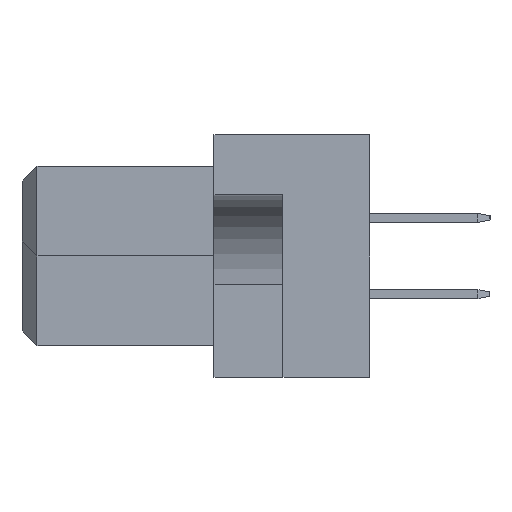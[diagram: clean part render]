
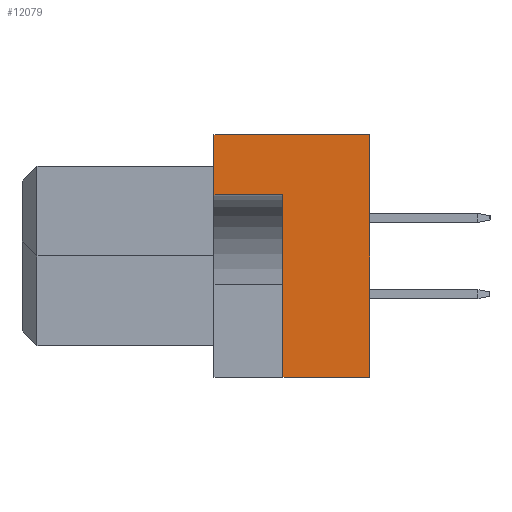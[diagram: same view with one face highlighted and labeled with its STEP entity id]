
A CAD part, left-side view. The second image highlights one B-rep face of the part: STEP entity #12079.
In plain terms, the highlighted planar face has unit normal (-1, 0, 0).
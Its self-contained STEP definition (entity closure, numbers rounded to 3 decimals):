
#908 = ORIENTED_EDGE ( 'NONE', *, *, #6201, .F. ) ;
#1047 = LINE ( 'NONE', #26575, #13743 ) ;
#1635 = VERTEX_POINT ( 'NONE', #16285 ) ;
#1842 = DIRECTION ( 'NONE',  ( 0., -1., 0. ) ) ;
#2089 = CARTESIAN_POINT ( 'NONE',  ( -47.5, 2.9, 2.05 ) ) ;
#2500 = CARTESIAN_POINT ( 'NONE',  ( -47.5, 0., 4.05 ) ) ;
#2769 = VERTEX_POINT ( 'NONE', #9849 ) ;
#2923 = VERTEX_POINT ( 'NONE', #15153 ) ;
#3946 = LINE ( 'NONE', #12339, #15631 ) ;
#4143 = DIRECTION ( 'NONE',  ( 0., 0., -1. ) ) ;
#4178 = DIRECTION ( 'NONE',  ( 0., 0., 1. ) ) ;
#4475 = VERTEX_POINT ( 'NONE', #8277 ) ;
#4609 = LINE ( 'NONE', #2500, #14750 ) ;
#4655 = FACE_OUTER_BOUND ( 'NONE', #23542, .T. ) ;
#6201 = EDGE_CURVE ( 'NONE', #27531, #4475, #25878, .T. ) ;
#6840 = LINE ( 'NONE', #2089, #27155 ) ;
#7661 = AXIS2_PLACEMENT_3D ( 'NONE', #14766, #19911, #4143 ) ;
#7951 = CARTESIAN_POINT ( 'NONE',  ( -47.5, 5.2, 4.05 ) ) ;
#8277 = CARTESIAN_POINT ( 'NONE',  ( -47.5, 0., 4.05 ) ) ;
#9849 = CARTESIAN_POINT ( 'NONE',  ( -47.5, 2.9, 2.05 ) ) ;
#11556 = EDGE_CURVE ( 'NONE', #2923, #27531, #18880, .T. ) ;
#12079 = ADVANCED_FACE ( 'NONE', ( #4655 ), #15290, .F. ) ;
#12339 = CARTESIAN_POINT ( 'NONE',  ( -47.5, 5.2, -4.05 ) ) ;
#13743 = VECTOR ( 'NONE', #15885, 1000. ) ;
#14356 = ORIENTED_EDGE ( 'NONE', *, *, #15703, .T. ) ;
#14566 = ORIENTED_EDGE ( 'NONE', *, *, #15091, .T. ) ;
#14750 = VECTOR ( 'NONE', #21560, 1000. ) ;
#14766 = CARTESIAN_POINT ( 'NONE',  ( -47.5, 5.2, 4.05 ) ) ;
#15091 = EDGE_CURVE ( 'NONE', #1635, #16895, #3946, .T. ) ;
#15153 = CARTESIAN_POINT ( 'NONE',  ( -47.5, 5.2, 2.05 ) ) ;
#15290 = PLANE ( 'NONE',  #7661 ) ;
#15631 = VECTOR ( 'NONE', #1842, 1000. ) ;
#15703 = EDGE_CURVE ( 'NONE', #16895, #4475, #4609, .T. ) ;
#15885 = DIRECTION ( 'NONE',  ( 0., 0., 1. ) ) ;
#16285 = CARTESIAN_POINT ( 'NONE',  ( -47.5, 2.9, -4.05 ) ) ;
#16895 = VERTEX_POINT ( 'NONE', #17355 ) ;
#17355 = CARTESIAN_POINT ( 'NONE',  ( -47.5, 0., -4.05 ) ) ;
#18880 = LINE ( 'NONE', #23360, #22401 ) ;
#19032 = DIRECTION ( 'NONE',  ( 0., 1., 0. ) ) ;
#19688 = CARTESIAN_POINT ( 'NONE',  ( -47.5, 5.2, 4.05 ) ) ;
#19911 = DIRECTION ( 'NONE',  ( 1., 0., 0. ) ) ;
#21541 = VECTOR ( 'NONE', #23615, 1000. ) ;
#21560 = DIRECTION ( 'NONE',  ( 0., 0., 1. ) ) ;
#22149 = ORIENTED_EDGE ( 'NONE', *, *, #25976, .F. ) ;
#22401 = VECTOR ( 'NONE', #4178, 1000. ) ;
#22615 = ORIENTED_EDGE ( 'NONE', *, *, #11556, .F. ) ;
#23360 = CARTESIAN_POINT ( 'NONE',  ( -47.5, 5.2, 4.05 ) ) ;
#23447 = ORIENTED_EDGE ( 'NONE', *, *, #24900, .F. ) ;
#23542 = EDGE_LOOP ( 'NONE', ( #22615, #22149, #23447, #14566, #14356, #908 ) ) ;
#23615 = DIRECTION ( 'NONE',  ( 0., -1., 0. ) ) ;
#24900 = EDGE_CURVE ( 'NONE', #1635, #2769, #1047, .T. ) ;
#25878 = LINE ( 'NONE', #19688, #21541 ) ;
#25976 = EDGE_CURVE ( 'NONE', #2769, #2923, #6840, .T. ) ;
#26575 = CARTESIAN_POINT ( 'NONE',  ( -47.5, 2.9, 2.05 ) ) ;
#27155 = VECTOR ( 'NONE', #19032, 1000. ) ;
#27531 = VERTEX_POINT ( 'NONE', #7951 ) ;
